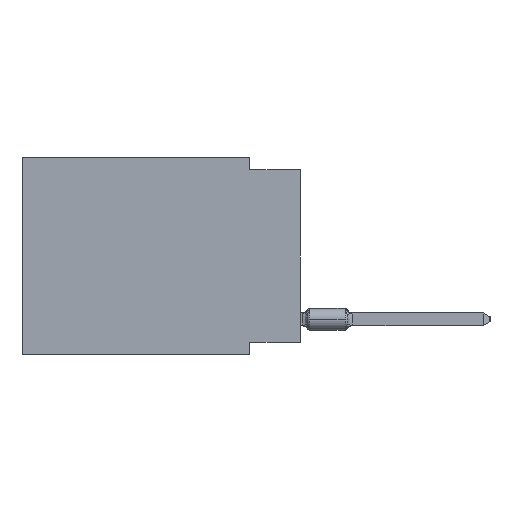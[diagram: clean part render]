
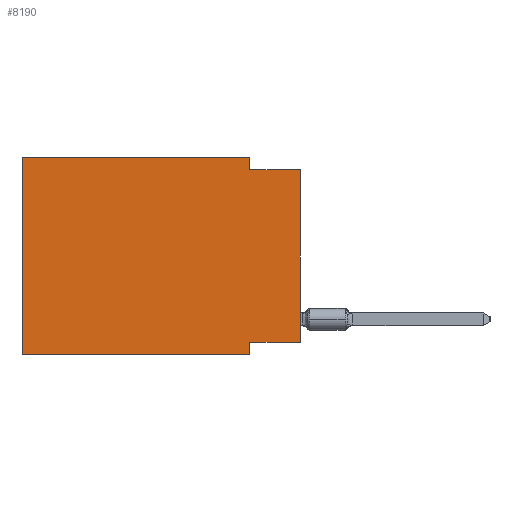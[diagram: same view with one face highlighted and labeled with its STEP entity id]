
A CAD part, left-side view. The second image highlights one B-rep face of the part: STEP entity #8190.
In plain terms, the highlighted planar face has unit normal (-1, 0, 0).
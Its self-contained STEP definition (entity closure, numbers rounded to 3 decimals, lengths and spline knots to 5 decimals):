
#1710 = VERTEX_POINT ( 'NONE', #78879 ) ;
#1921 = CARTESIAN_POINT ( 'NONE',  ( 0., 0.55, 0. ) ) ;
#2242 = FACE_OUTER_BOUND ( 'NONE', #36840, .T. ) ;
#3710 = CARTESIAN_POINT ( 'NONE',  ( 0., 0.1, -0.365 ) ) ;
#7141 = DIRECTION ( 'NONE',  ( 0., 0., 1. ) ) ;
#8190 = ADVANCED_FACE ( 'NONE', ( #2242 ), #27691, .F. ) ;
#8199 = CARTESIAN_POINT ( 'NONE',  ( 0., 0.55, -0.39 ) ) ;
#10729 = VECTOR ( 'NONE', #80876, 39.37008 ) ;
#13292 = AXIS2_PLACEMENT_3D ( 'NONE', #39210, #77840, #40839 ) ;
#13865 = DIRECTION ( 'NONE',  ( 0., -1., 0. ) ) ;
#17413 = ORIENTED_EDGE ( 'NONE', *, *, #67742, .T. ) ;
#17904 = VERTEX_POINT ( 'NONE', #8199 ) ;
#19615 = CARTESIAN_POINT ( 'NONE',  ( 0., 0., -0.025 ) ) ;
#22231 = VECTOR ( 'NONE', #41778, 39.37008 ) ;
#24466 = CARTESIAN_POINT ( 'NONE',  ( 0., 0.55, 0. ) ) ;
#24960 = CARTESIAN_POINT ( 'NONE',  ( 0., 0.55, 0. ) ) ;
#25821 = VERTEX_POINT ( 'NONE', #1921 ) ;
#26435 = LINE ( 'NONE', #44151, #72367 ) ;
#27531 = CARTESIAN_POINT ( 'NONE',  ( 0., 0.1, -0.025 ) ) ;
#27691 = PLANE ( 'NONE',  #13292 ) ;
#28897 = VERTEX_POINT ( 'NONE', #31399 ) ;
#28988 = ORIENTED_EDGE ( 'NONE', *, *, #78370, .F. ) ;
#30507 = LINE ( 'NONE', #42856, #46026 ) ;
#31399 = CARTESIAN_POINT ( 'NONE',  ( 0., 0.1, 0. ) ) ;
#31451 = DIRECTION ( 'NONE',  ( 0., 0., 1. ) ) ;
#32245 = VECTOR ( 'NONE', #32556, 39.37008 ) ;
#32556 = DIRECTION ( 'NONE',  ( 0., -1., 0. ) ) ;
#33105 = VECTOR ( 'NONE', #60855, 39.37008 ) ;
#34684 = VERTEX_POINT ( 'NONE', #49912 ) ;
#35202 = LINE ( 'NONE', #60295, #22231 ) ;
#35861 = DIRECTION ( 'NONE',  ( 0., 0., -1. ) ) ;
#36840 = EDGE_LOOP ( 'NONE', ( #63694, #53059, #64296, #28988, #46011, #17413, #76459, #63349 ) ) ;
#39210 = CARTESIAN_POINT ( 'NONE',  ( 0., 0.55, 0. ) ) ;
#40839 = DIRECTION ( 'NONE',  ( 0., 0., -1. ) ) ;
#40856 = EDGE_CURVE ( 'NONE', #28897, #66113, #35202, .T. ) ;
#41560 = LINE ( 'NONE', #60078, #33105 ) ;
#41778 = DIRECTION ( 'NONE',  ( 0., 0., -1. ) ) ;
#42704 = EDGE_CURVE ( 'NONE', #34684, #44475, #26435, .T. ) ;
#42856 = CARTESIAN_POINT ( 'NONE',  ( 0., 0.1, -0.39 ) ) ;
#44151 = CARTESIAN_POINT ( 'NONE',  ( 0., 0., 0. ) ) ;
#44475 = VERTEX_POINT ( 'NONE', #79587 ) ;
#46011 = ORIENTED_EDGE ( 'NONE', *, *, #52385, .F. ) ;
#46026 = VECTOR ( 'NONE', #35861, 39.37008 ) ;
#49912 = CARTESIAN_POINT ( 'NONE',  ( 0., 0., -0.365 ) ) ;
#51068 = CARTESIAN_POINT ( 'NONE',  ( 0., 0.55, -0.39 ) ) ;
#52385 = EDGE_CURVE ( 'NONE', #17904, #25821, #62703, .T. ) ;
#53059 = ORIENTED_EDGE ( 'NONE', *, *, #59569, .F. ) ;
#55808 = LINE ( 'NONE', #24960, #10729 ) ;
#57983 = VECTOR ( 'NONE', #13865, 39.37008 ) ;
#59569 = EDGE_CURVE ( 'NONE', #66113, #44475, #69755, .T. ) ;
#60076 = EDGE_CURVE ( 'NONE', #34684, #71351, #41560, .T. ) ;
#60078 = CARTESIAN_POINT ( 'NONE',  ( 0., 0., -0.365 ) ) ;
#60295 = CARTESIAN_POINT ( 'NONE',  ( 0., 0.1, 0. ) ) ;
#60855 = DIRECTION ( 'NONE',  ( 0., 1., 0. ) ) ;
#62703 = LINE ( 'NONE', #24466, #71808 ) ;
#62990 = LINE ( 'NONE', #51068, #32245 ) ;
#63349 = ORIENTED_EDGE ( 'NONE', *, *, #60076, .F. ) ;
#63694 = ORIENTED_EDGE ( 'NONE', *, *, #42704, .T. ) ;
#64296 = ORIENTED_EDGE ( 'NONE', *, *, #40856, .F. ) ;
#66113 = VERTEX_POINT ( 'NONE', #27531 ) ;
#67742 = EDGE_CURVE ( 'NONE', #17904, #1710, #62990, .T. ) ;
#69755 = LINE ( 'NONE', #19615, #57983 ) ;
#71351 = VERTEX_POINT ( 'NONE', #3710 ) ;
#71808 = VECTOR ( 'NONE', #31451, 39.37008 ) ;
#72367 = VECTOR ( 'NONE', #7141, 39.37008 ) ;
#76459 = ORIENTED_EDGE ( 'NONE', *, *, #76861, .F. ) ;
#76861 = EDGE_CURVE ( 'NONE', #71351, #1710, #30507, .T. ) ;
#77840 = DIRECTION ( 'NONE',  ( 1., 0., 0. ) ) ;
#78370 = EDGE_CURVE ( 'NONE', #25821, #28897, #55808, .T. ) ;
#78879 = CARTESIAN_POINT ( 'NONE',  ( 0., 0.1, -0.39 ) ) ;
#79587 = CARTESIAN_POINT ( 'NONE',  ( 0., 0., -0.025 ) ) ;
#80876 = DIRECTION ( 'NONE',  ( 0., -1., 0. ) ) ;
